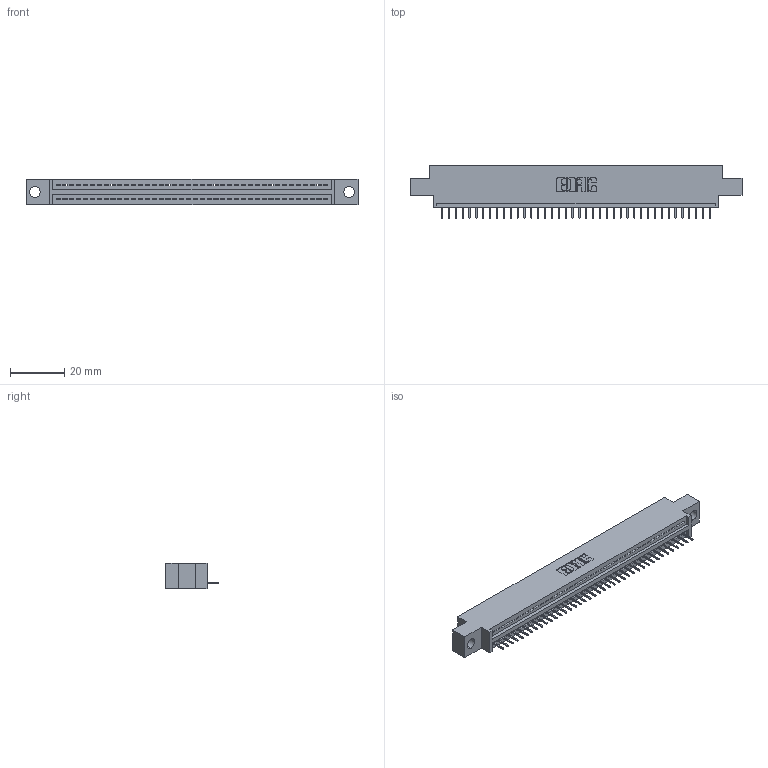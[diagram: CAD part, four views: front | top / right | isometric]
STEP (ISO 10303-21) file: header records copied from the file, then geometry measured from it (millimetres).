
FILE_DESCRIPTION (( 'STEP AP203' ), '1' );
FILE_NAME ('345-040-524-604.STEP', '2018-09-05T02:37:51', ( '' ), ( '' ), 'SwSTEP 2.0', 'SolidWorks 2016', '' );
FILE_SCHEMA (( 'CONFIG_CONTROL_DESIGN' ));
Length unit declared in the file: inch
Products named in the file (3): 345 Part_0.170 Offset - 0.156 Dia-TH; 345-292-001_345-293-124; 345-040-524-604
Assembly tree (41 placements, depth 2):
  345-040-524-604
    345 Part_0.170 Offset - 0.156 Dia-TH
    345-292-001_345-293-124  x40
Bounding box: 122.81 x 19.35 x 9.4 mm (x, y, z)
Volume: 11288.9 mm3; surface area: 14404.8 mm2
Topology: 41 solids, 41 shells, 2610 faces, 7553 edges, 4874 vertices
Faces by surface type: plane 1924, cylinder 686
Entity records: 30583 total; most frequent: CARTESIAN_POINT 5304, ORIENTED_EDGE 5278, DIRECTION 4635, EDGE_CURVE 2639, VECTOR 2351, LINE 2351, VERTEX_POINT 1754, AXIS2_PLACEMENT_3D 1142
